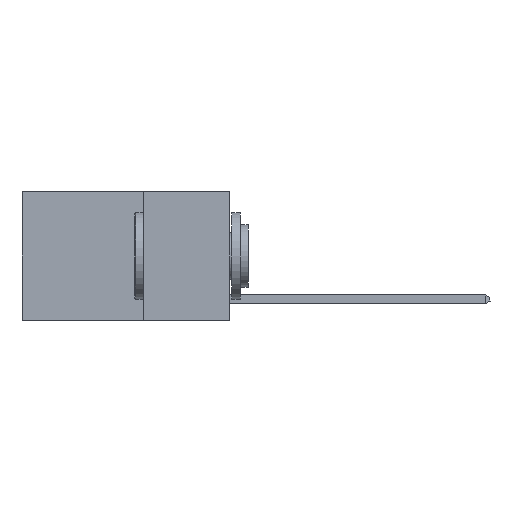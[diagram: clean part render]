
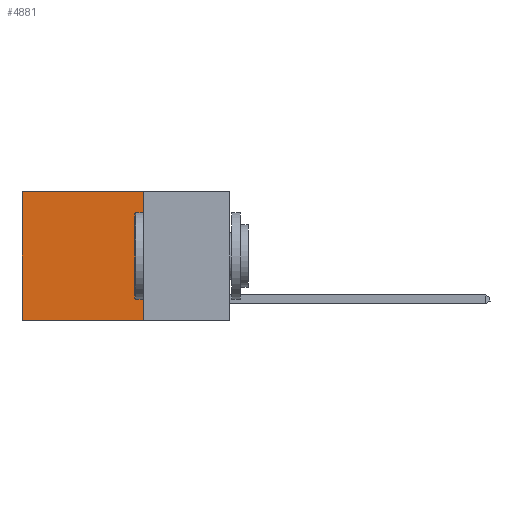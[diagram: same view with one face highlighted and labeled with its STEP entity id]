
A CAD part, left-side view. The second image highlights one B-rep face of the part: STEP entity #4881.
In plain terms, the highlighted planar face has unit normal (-1, 0, 0).
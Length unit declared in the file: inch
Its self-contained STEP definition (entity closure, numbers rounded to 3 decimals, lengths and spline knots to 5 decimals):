
#561 = VERTEX_POINT ( 'NONE', #17518 ) ;
#1439 = DIRECTION ( 'NONE',  ( 0., 1., 0. ) ) ;
#1879 = EDGE_CURVE ( 'NONE', #561, #12034, #9254, .T. ) ;
#2376 = VERTEX_POINT ( 'NONE', #30062 ) ;
#3649 = VECTOR ( 'NONE', #1439, 39.37008 ) ;
#4344 = CARTESIAN_POINT ( 'NONE',  ( 0.2625, 0.25, 0. ) ) ;
#4881 = ADVANCED_FACE ( 'NONE', ( #7556 ), #24801, .F. ) ;
#6016 = DIRECTION ( 'NONE',  ( 0., 0., -1. ) ) ;
#6021 = EDGE_CURVE ( 'NONE', #27327, #2376, #28598, .T. ) ;
#7031 = VECTOR ( 'NONE', #8919, 39.37008 ) ;
#7556 = FACE_OUTER_BOUND ( 'NONE', #13517, .T. ) ;
#7885 = CARTESIAN_POINT ( 'NONE',  ( 0.2625, 0.25, 0. ) ) ;
#8039 = VECTOR ( 'NONE', #12101, 39.37008 ) ;
#8572 = CARTESIAN_POINT ( 'NONE',  ( 0.2625, 0.25, -0.37 ) ) ;
#8919 = DIRECTION ( 'NONE',  ( 0., 0., -1. ) ) ;
#9254 = LINE ( 'NONE', #11185, #7031 ) ;
#11185 = CARTESIAN_POINT ( 'NONE',  ( 0.2625, 0.6, 0. ) ) ;
#12034 = VERTEX_POINT ( 'NONE', #12619 ) ;
#12101 = DIRECTION ( 'NONE',  ( 0., 1., 0. ) ) ;
#12619 = CARTESIAN_POINT ( 'NONE',  ( 0.2625, 0.6, -0.37 ) ) ;
#12709 = CARTESIAN_POINT ( 'NONE',  ( 0.2625, 0.25, 0. ) ) ;
#12825 = LINE ( 'NONE', #16594, #8039 ) ;
#13517 = EDGE_LOOP ( 'NONE', ( #17228, #29824, #18660, #18449 ) ) ;
#13856 = DIRECTION ( 'NONE',  ( 0., 0., -1. ) ) ;
#14524 = VECTOR ( 'NONE', #13856, 39.37008 ) ;
#16594 = CARTESIAN_POINT ( 'NONE',  ( 0.2625, 0.25, 0. ) ) ;
#16998 = LINE ( 'NONE', #8572, #3649 ) ;
#17228 = ORIENTED_EDGE ( 'NONE', *, *, #1879, .T. ) ;
#17518 = CARTESIAN_POINT ( 'NONE',  ( 0.2625, 0.6, 0. ) ) ;
#18449 = ORIENTED_EDGE ( 'NONE', *, *, #25672, .T. ) ;
#18660 = ORIENTED_EDGE ( 'NONE', *, *, #6021, .F. ) ;
#22895 = EDGE_CURVE ( 'NONE', #2376, #12034, #16998, .T. ) ;
#23240 = AXIS2_PLACEMENT_3D ( 'NONE', #12709, #29564, #6016 ) ;
#24801 = PLANE ( 'NONE',  #23240 ) ;
#25672 = EDGE_CURVE ( 'NONE', #27327, #561, #12825, .T. ) ;
#27327 = VERTEX_POINT ( 'NONE', #7885 ) ;
#28598 = LINE ( 'NONE', #4344, #14524 ) ;
#29564 = DIRECTION ( 'NONE',  ( 1., 0., 0. ) ) ;
#29824 = ORIENTED_EDGE ( 'NONE', *, *, #22895, .F. ) ;
#30062 = CARTESIAN_POINT ( 'NONE',  ( 0.2625, 0.25, -0.37 ) ) ;
